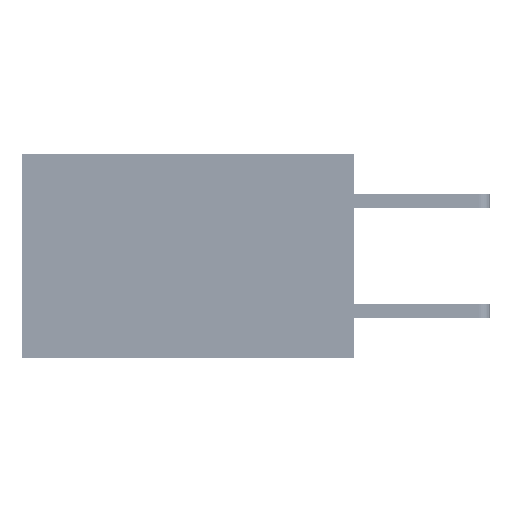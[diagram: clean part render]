
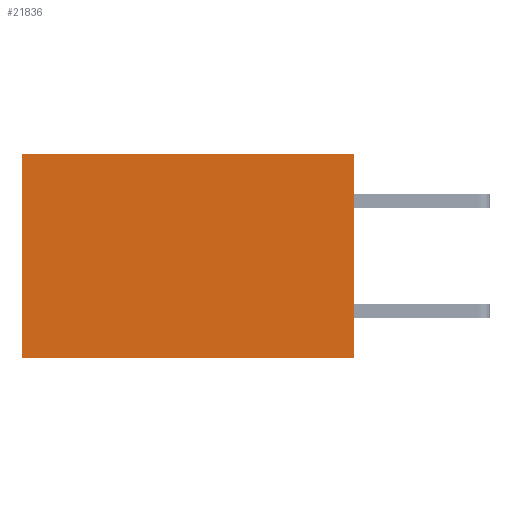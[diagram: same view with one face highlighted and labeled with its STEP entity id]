
A CAD part, left-side view. The second image highlights one B-rep face of the part: STEP entity #21836.
In plain terms, the highlighted planar face has unit normal (-1, 0, 0).
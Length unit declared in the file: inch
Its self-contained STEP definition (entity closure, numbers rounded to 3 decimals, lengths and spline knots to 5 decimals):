
#255 = VECTOR ( 'NONE', #24954, 39.37008 ) ;
#737 = DIRECTION ( 'NONE',  ( 0., 1., 0. ) ) ;
#971 = CARTESIAN_POINT ( 'NONE',  ( 0.2875, 0., 0. ) ) ;
#1750 = CARTESIAN_POINT ( 'NONE',  ( 0.2875, 0., 0. ) ) ;
#2522 = ORIENTED_EDGE ( 'NONE', *, *, #32896, .F. ) ;
#3462 = VECTOR ( 'NONE', #30799, 39.37008 ) ;
#4555 = VECTOR ( 'NONE', #19097, 39.37008 ) ;
#5009 = LINE ( 'NONE', #33629, #4555 ) ;
#8877 = CARTESIAN_POINT ( 'NONE',  ( 0.2875, 0., 0. ) ) ;
#10184 = LINE ( 'NONE', #45581, #255 ) ;
#11016 = VERTEX_POINT ( 'NONE', #30944 ) ;
#15287 = VERTEX_POINT ( 'NONE', #38740 ) ;
#17632 = CARTESIAN_POINT ( 'NONE',  ( 0.2875, 0., 0. ) ) ;
#18418 = ORIENTED_EDGE ( 'NONE', *, *, #20405, .F. ) ;
#19097 = DIRECTION ( 'NONE',  ( 0., 0., -1. ) ) ;
#19702 = VERTEX_POINT ( 'NONE', #971 ) ;
#20129 = FACE_OUTER_BOUND ( 'NONE', #29261, .T. ) ;
#20350 = DIRECTION ( 'NONE',  ( 0., 0., -1. ) ) ;
#20405 = EDGE_CURVE ( 'NONE', #32622, #11016, #10184, .T. ) ;
#21248 = ORIENTED_EDGE ( 'NONE', *, *, #38311, .T. ) ;
#21836 = ADVANCED_FACE ( 'NONE', ( #20129 ), #26936, .F. ) ;
#22083 = VECTOR ( 'NONE', #737, 39.37008 ) ;
#22861 = CARTESIAN_POINT ( 'NONE',  ( 0.2875, 0., -0.37 ) ) ;
#24954 = DIRECTION ( 'NONE',  ( 0., 1., 0. ) ) ;
#26429 = AXIS2_PLACEMENT_3D ( 'NONE', #8877, #44952, #20350 ) ;
#26936 = PLANE ( 'NONE',  #26429 ) ;
#29261 = EDGE_LOOP ( 'NONE', ( #21248, #18418, #2522, #40085 ) ) ;
#30799 = DIRECTION ( 'NONE',  ( 0., 0., -1. ) ) ;
#30944 = CARTESIAN_POINT ( 'NONE',  ( 0.2875, 0.6, -0.37 ) ) ;
#32622 = VERTEX_POINT ( 'NONE', #22861 ) ;
#32896 = EDGE_CURVE ( 'NONE', #19702, #32622, #34777, .T. ) ;
#33629 = CARTESIAN_POINT ( 'NONE',  ( 0.2875, 0.6, 0. ) ) ;
#34777 = LINE ( 'NONE', #1750, #3462 ) ;
#38311 = EDGE_CURVE ( 'NONE', #15287, #11016, #5009, .T. ) ;
#38740 = CARTESIAN_POINT ( 'NONE',  ( 0.2875, 0.6, 0. ) ) ;
#40085 = ORIENTED_EDGE ( 'NONE', *, *, #42509, .T. ) ;
#42509 = EDGE_CURVE ( 'NONE', #19702, #15287, #46215, .T. ) ;
#44952 = DIRECTION ( 'NONE',  ( 1., 0., 0. ) ) ;
#45581 = CARTESIAN_POINT ( 'NONE',  ( 0.2875, 0., -0.37 ) ) ;
#46215 = LINE ( 'NONE', #17632, #22083 ) ;
